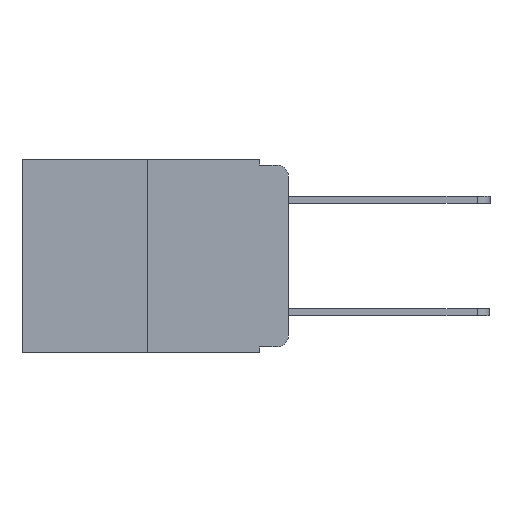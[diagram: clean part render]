
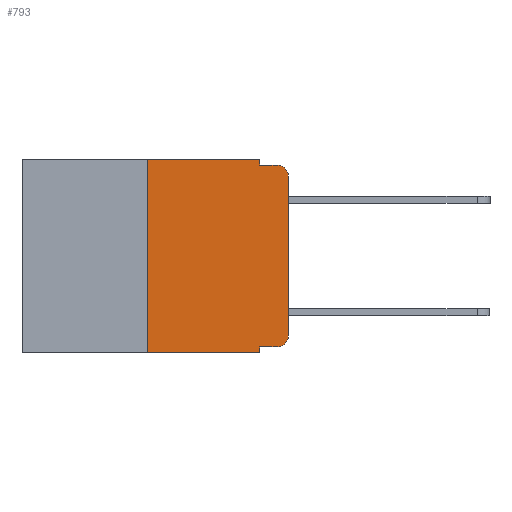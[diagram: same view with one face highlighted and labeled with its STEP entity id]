
A CAD part, left-side view. The second image highlights one B-rep face of the part: STEP entity #793.
In plain terms, the highlighted planar face has unit normal (-1, 0, 0).
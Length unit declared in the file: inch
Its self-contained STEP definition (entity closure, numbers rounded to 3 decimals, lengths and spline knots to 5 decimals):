
#63 = ORIENTED_EDGE ( 'NONE', *, *, #2514, .T. ) ;
#120 = ORIENTED_EDGE ( 'NONE', *, *, #5599, .F. ) ;
#242 = EDGE_CURVE ( 'NONE', #8310, #5036, #8170, .T. ) ;
#301 = VERTEX_POINT ( 'NONE', #9137 ) ;
#319 = VERTEX_POINT ( 'NONE', #5702 ) ;
#333 = ORIENTED_EDGE ( 'NONE', *, *, #5727, .T. ) ;
#433 = ORIENTED_EDGE ( 'NONE', *, *, #7328, .T. ) ;
#561 = LINE ( 'NONE', #5403, #2600 ) ;
#793 = ADVANCED_FACE ( 'NONE', ( #2398 ), #6483, .F. ) ;
#801 = CARTESIAN_POINT ( 'NONE',  ( 0., 0.25, -0.343 ) ) ;
#1006 = CARTESIAN_POINT ( 'NONE',  ( 0., 0.051, -0.343 ) ) ;
#1094 = CARTESIAN_POINT ( 'NONE',  ( 0., 0., -0.03 ) ) ;
#1219 = VECTOR ( 'NONE', #3691, 39.37008 ) ;
#1485 = DIRECTION ( 'NONE',  ( 0., -1., 0. ) ) ;
#1508 = VECTOR ( 'NONE', #7100, 39.37008 ) ;
#1569 = ORIENTED_EDGE ( 'NONE', *, *, #2617, .T. ) ;
#1683 = DIRECTION ( 'NONE',  ( 0., 0., -1. ) ) ;
#1838 = EDGE_CURVE ( 'NONE', #319, #301, #7177, .T. ) ;
#1855 = VECTOR ( 'NONE', #8874, 39.37008 ) ;
#1878 = ORIENTED_EDGE ( 'NONE', *, *, #242, .T. ) ;
#1914 = CARTESIAN_POINT ( 'NONE',  ( 0., 0., -0.313 ) ) ;
#2027 = ORIENTED_EDGE ( 'NONE', *, *, #4580, .F. ) ;
#2241 = AXIS2_PLACEMENT_3D ( 'NONE', #8007, #3670, #8691 ) ;
#2343 = DIRECTION ( 'NONE',  ( 0., -1., 0. ) ) ;
#2377 = VERTEX_POINT ( 'NONE', #10199 ) ;
#2398 = FACE_OUTER_BOUND ( 'NONE', #9989, .T. ) ;
#2441 = DIRECTION ( 'NONE',  ( 1., 0., 0. ) ) ;
#2514 = EDGE_CURVE ( 'NONE', #6130, #8262, #5034, .T. ) ;
#2600 = VECTOR ( 'NONE', #1485, 39.37008 ) ;
#2617 = EDGE_CURVE ( 'NONE', #5199, #8310, #7707, .T. ) ;
#2929 = ORIENTED_EDGE ( 'NONE', *, *, #2954, .F. ) ;
#2954 = EDGE_CURVE ( 'NONE', #301, #7341, #8233, .T. ) ;
#2960 = CARTESIAN_POINT ( 'NONE',  ( 0., 0., 0. ) ) ;
#3670 = DIRECTION ( 'NONE',  ( -1., 0., 0. ) ) ;
#3691 = DIRECTION ( 'NONE',  ( 0., 0., -1. ) ) ;
#3880 = ORIENTED_EDGE ( 'NONE', *, *, #1838, .F. ) ;
#4001 = CARTESIAN_POINT ( 'NONE',  ( 0., 0.051, -0.333 ) ) ;
#4021 = CARTESIAN_POINT ( 'NONE',  ( 0., 0.473, 0. ) ) ;
#4193 = LINE ( 'NONE', #8799, #1855 ) ;
#4231 = ORIENTED_EDGE ( 'NONE', *, *, #6085, .F. ) ;
#4410 = DIRECTION ( 'NONE',  ( 0., 0., -1. ) ) ;
#4459 = CARTESIAN_POINT ( 'NONE',  ( 0., 0.051, -0.01 ) ) ;
#4580 = EDGE_CURVE ( 'NONE', #7341, #5036, #9551, .T. ) ;
#4619 = AXIS2_PLACEMENT_3D ( 'NONE', #4021, #2441, #4410 ) ;
#5034 = LINE ( 'NONE', #6741, #8765 ) ;
#5036 = VERTEX_POINT ( 'NONE', #6702 ) ;
#5110 = CARTESIAN_POINT ( 'NONE',  ( 0., 0.051, 0. ) ) ;
#5158 = AXIS2_PLACEMENT_3D ( 'NONE', #10118, #5319, #1683 ) ;
#5199 = VERTEX_POINT ( 'NONE', #1914 ) ;
#5219 = CIRCLE ( 'NONE', #2241, 0.02 ) ;
#5292 = VECTOR ( 'NONE', #10060, 39.37008 ) ;
#5319 = DIRECTION ( 'NONE',  ( -1., 0., 0. ) ) ;
#5403 = CARTESIAN_POINT ( 'NONE',  ( 0., 0.051, -0.333 ) ) ;
#5599 = EDGE_CURVE ( 'NONE', #5664, #8262, #7568, .T. ) ;
#5664 = VERTEX_POINT ( 'NONE', #4001 ) ;
#5702 = CARTESIAN_POINT ( 'NONE',  ( 0., 0.25, 0. ) ) ;
#5727 = EDGE_CURVE ( 'NONE', #5664, #2377, #561, .T. ) ;
#6085 = EDGE_CURVE ( 'NONE', #6130, #319, #4193, .T. ) ;
#6130 = VERTEX_POINT ( 'NONE', #801 ) ;
#6136 = CARTESIAN_POINT ( 'NONE',  ( 0., 0.051, 0. ) ) ;
#6146 = DIRECTION ( 'NONE',  ( 0., 0., -1. ) ) ;
#6232 = CARTESIAN_POINT ( 'NONE',  ( 0., 0.051, -0.01 ) ) ;
#6483 = PLANE ( 'NONE',  #4619 ) ;
#6702 = CARTESIAN_POINT ( 'NONE',  ( 0., 0.02, -0.01 ) ) ;
#6741 = CARTESIAN_POINT ( 'NONE',  ( 0., 0.473, -0.343 ) ) ;
#7100 = DIRECTION ( 'NONE',  ( 0., -1., 0. ) ) ;
#7177 = LINE ( 'NONE', #9995, #5292 ) ;
#7328 = EDGE_CURVE ( 'NONE', #2377, #5199, #5219, .T. ) ;
#7341 = VERTEX_POINT ( 'NONE', #4459 ) ;
#7568 = LINE ( 'NONE', #5110, #1219 ) ;
#7707 = LINE ( 'NONE', #2960, #9484 ) ;
#7786 = DIRECTION ( 'NONE',  ( 0., 0., 1. ) ) ;
#8007 = CARTESIAN_POINT ( 'NONE',  ( 0., 0.02, -0.313 ) ) ;
#8017 = VECTOR ( 'NONE', #6146, 39.37008 ) ;
#8170 = CIRCLE ( 'NONE', #5158, 0.02 ) ;
#8233 = LINE ( 'NONE', #6136, #8017 ) ;
#8262 = VERTEX_POINT ( 'NONE', #1006 ) ;
#8310 = VERTEX_POINT ( 'NONE', #1094 ) ;
#8691 = DIRECTION ( 'NONE',  ( 0., 0., -1. ) ) ;
#8765 = VECTOR ( 'NONE', #2343, 39.37008 ) ;
#8799 = CARTESIAN_POINT ( 'NONE',  ( 0., 0.25, 0. ) ) ;
#8874 = DIRECTION ( 'NONE',  ( 0., 0., 1. ) ) ;
#9137 = CARTESIAN_POINT ( 'NONE',  ( 0., 0.051, 0. ) ) ;
#9484 = VECTOR ( 'NONE', #7786, 39.37008 ) ;
#9551 = LINE ( 'NONE', #6232, #1508 ) ;
#9989 = EDGE_LOOP ( 'NONE', ( #1569, #1878, #2027, #2929, #3880, #4231, #63, #120, #333, #433 ) ) ;
#9995 = CARTESIAN_POINT ( 'NONE',  ( 0., 0.473, 0. ) ) ;
#10060 = DIRECTION ( 'NONE',  ( 0., -1., 0. ) ) ;
#10118 = CARTESIAN_POINT ( 'NONE',  ( 0., 0.02, -0.03 ) ) ;
#10199 = CARTESIAN_POINT ( 'NONE',  ( 0., 0.02, -0.333 ) ) ;
